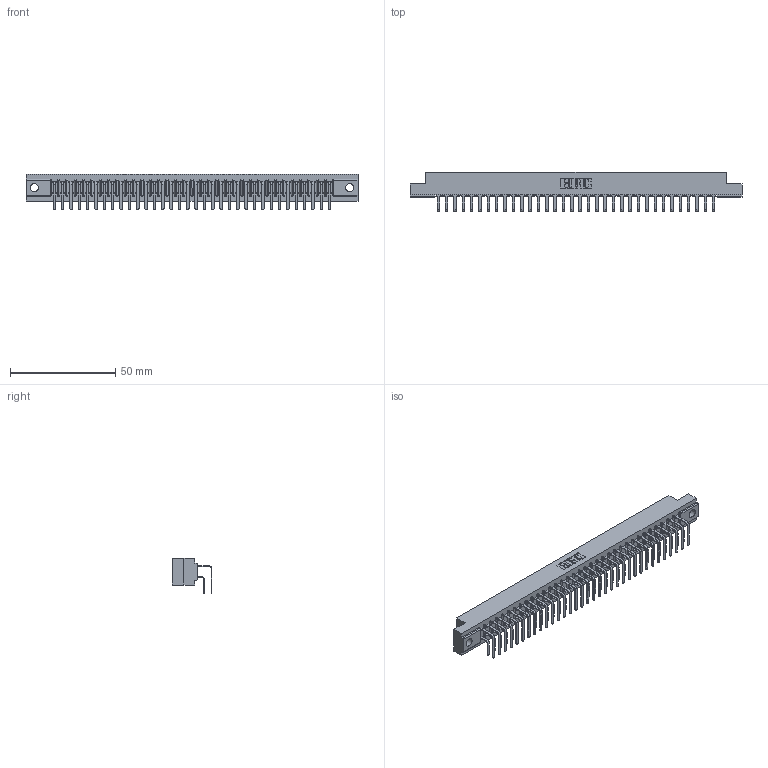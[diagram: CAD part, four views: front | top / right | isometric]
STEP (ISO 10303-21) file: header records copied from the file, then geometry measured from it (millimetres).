
FILE_DESCRIPTION (( 'STEP AP203' ), '1' );
FILE_NAME ('357-034-558-104.STEP', '2018-08-10T02:16:46', ( '' ), ( '' ), 'SwSTEP 2.0', 'SolidWorks 2016', '' );
FILE_SCHEMA (( 'CONFIG_CONTROL_DESIGN' ));
Length unit declared in the file: inch
Products named in the file (4): 307-290-001_558 - 2 (Single); 357-034-558-104; 307 Part_.156 Dia Mounting Holes; 307-290-001_558 559 - 1 (Single)
Assembly tree (69 placements, depth 2):
  357-034-558-104
    307 Part_.156 Dia Mounting Holes
    307-290-001_558 559 - 1 (Single)  x34
    307-290-001_558 - 2 (Single)  x34
Bounding box: 157.73 x 18.96 x 16.8 mm (x, y, z)
Volume: 16912 mm3; surface area: 22120.9 mm2
Topology: 69 solids, 69 shells, 3567 faces, 10015 edges, 6490 vertices
Faces by surface type: plane 2328, cylinder 1169, sphere 70
Entity records: 33087 total; most frequent: CARTESIAN_POINT 5422, ORIENTED_EDGE 5370, DIRECTION 5305, EDGE_CURVE 2685, VECTOR 2063, LINE 2063, VERTEX_POINT 1738, AXIS2_PLACEMENT_3D 1621
